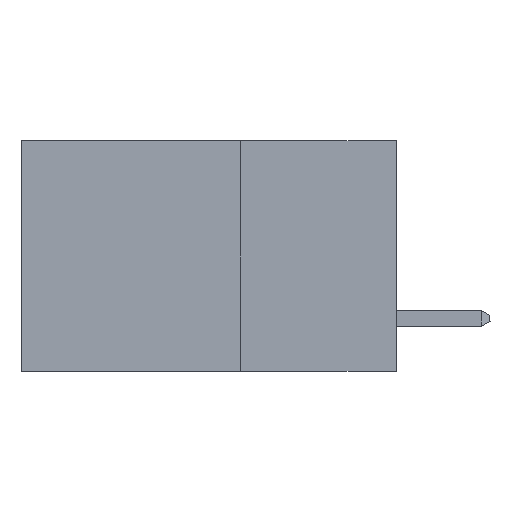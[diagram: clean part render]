
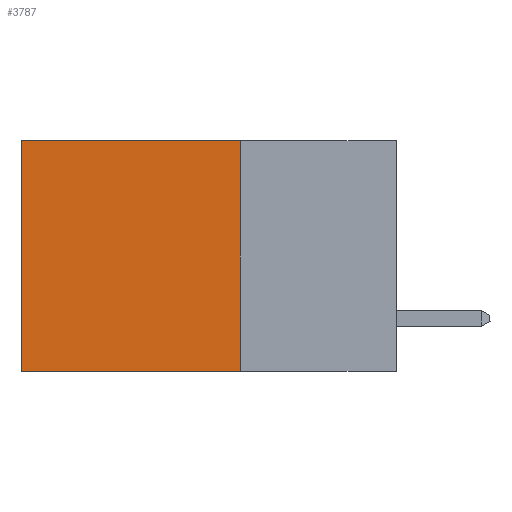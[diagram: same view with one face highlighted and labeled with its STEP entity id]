
A CAD part, left-side view. The second image highlights one B-rep face of the part: STEP entity #3787.
In plain terms, the highlighted planar face has unit normal (-1, 0, 0).
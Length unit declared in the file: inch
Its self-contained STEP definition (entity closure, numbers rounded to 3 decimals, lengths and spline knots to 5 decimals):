
#46 = DIRECTION ( 'NONE',  ( 0., 1., 0. ) ) ;
#70 = AXIS2_PLACEMENT_3D ( 'NONE', #4430, #889, #10980 ) ;
#75 = ORIENTED_EDGE ( 'NONE', *, *, #13221, .F. ) ;
#93 = CARTESIAN_POINT ( 'NONE',  ( 0.2615, 0.25, -0.37 ) ) ;
#215 = CARTESIAN_POINT ( 'NONE',  ( 0.2615, 0.6, -0.37 ) ) ;
#335 = LINE ( 'NONE', #10364, #8507 ) ;
#419 = CARTESIAN_POINT ( 'NONE',  ( 0.2615, 0.6, -0.37 ) ) ;
#889 = DIRECTION ( 'NONE',  ( 1., 0., 0. ) ) ;
#1153 = CARTESIAN_POINT ( 'NONE',  ( 0.2615, 0.25, -0.37 ) ) ;
#2299 = CARTESIAN_POINT ( 'NONE',  ( 0.2615, 0.6, 0. ) ) ;
#3031 = VECTOR ( 'NONE', #12709, 39.37008 ) ;
#3039 = VERTEX_POINT ( 'NONE', #2299 ) ;
#3339 = EDGE_CURVE ( 'NONE', #3039, #11320, #9764, .T. ) ;
#3394 = VECTOR ( 'NONE', #8614, 39.37008 ) ;
#3522 = DIRECTION ( 'NONE',  ( 0., 1., 0. ) ) ;
#3787 = ADVANCED_FACE ( 'NONE', ( #14125 ), #5510, .F. ) ;
#4061 = LINE ( 'NONE', #1153, #4624 ) ;
#4430 = CARTESIAN_POINT ( 'NONE',  ( 0.2615, 0.25, -0.37 ) ) ;
#4624 = VECTOR ( 'NONE', #46, 39.37008 ) ;
#5510 = PLANE ( 'NONE',  #70 ) ;
#6187 = LINE ( 'NONE', #12612, #3031 ) ;
#6918 = EDGE_CURVE ( 'NONE', #7324, #3039, #335, .T. ) ;
#7324 = VERTEX_POINT ( 'NONE', #10142 ) ;
#8179 = EDGE_CURVE ( 'NONE', #7324, #11581, #6187, .T. ) ;
#8507 = VECTOR ( 'NONE', #3522, 39.37008 ) ;
#8614 = DIRECTION ( 'NONE',  ( 0., 0., -1. ) ) ;
#9764 = LINE ( 'NONE', #419, #3394 ) ;
#10142 = CARTESIAN_POINT ( 'NONE',  ( 0.2615, 0.25, 0. ) ) ;
#10364 = CARTESIAN_POINT ( 'NONE',  ( 0.2615, 0.25, 0. ) ) ;
#10980 = DIRECTION ( 'NONE',  ( 0., 0., -1. ) ) ;
#11320 = VERTEX_POINT ( 'NONE', #215 ) ;
#11581 = VERTEX_POINT ( 'NONE', #93 ) ;
#11660 = EDGE_LOOP ( 'NONE', ( #14640, #75, #11964, #11837 ) ) ;
#11837 = ORIENTED_EDGE ( 'NONE', *, *, #6918, .T. ) ;
#11964 = ORIENTED_EDGE ( 'NONE', *, *, #8179, .F. ) ;
#12612 = CARTESIAN_POINT ( 'NONE',  ( 0.2615, 0.25, -0.37 ) ) ;
#12709 = DIRECTION ( 'NONE',  ( 0., 0., -1. ) ) ;
#13221 = EDGE_CURVE ( 'NONE', #11581, #11320, #4061, .T. ) ;
#14125 = FACE_OUTER_BOUND ( 'NONE', #11660, .T. ) ;
#14640 = ORIENTED_EDGE ( 'NONE', *, *, #3339, .T. ) ;
